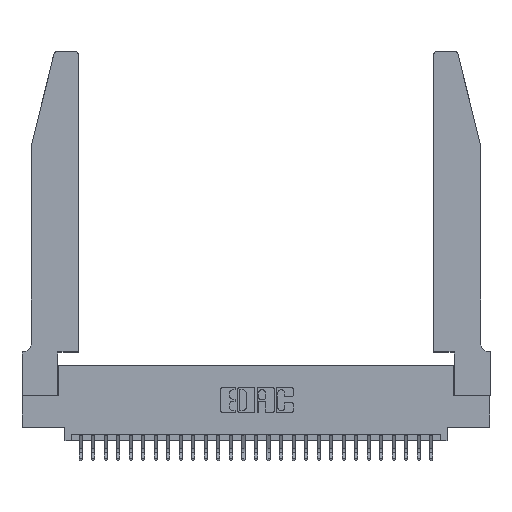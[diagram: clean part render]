
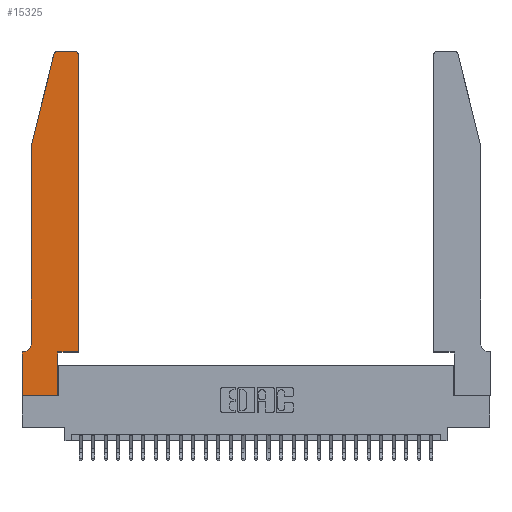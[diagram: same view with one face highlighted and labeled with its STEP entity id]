
A CAD part, top view. The second image highlights one B-rep face of the part: STEP entity #15325.
In plain terms, the highlighted planar face has unit normal (0, 0, 1).
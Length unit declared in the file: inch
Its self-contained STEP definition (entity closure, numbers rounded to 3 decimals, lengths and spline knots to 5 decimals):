
#506 = CARTESIAN_POINT ( 'NONE',  ( 0., 0., 0.37 ) ) ;
#658 = DIRECTION ( 'NONE',  ( -1., 0., 0. ) ) ;
#1285 = VECTOR ( 'NONE', #10921, 39.37008 ) ;
#1309 = ORIENTED_EDGE ( 'NONE', *, *, #6473, .T. ) ;
#1314 = CARTESIAN_POINT ( 'NONE',  ( 0.4505, 0.35, 0.37 ) ) ;
#1376 = CARTESIAN_POINT ( 'NONE',  ( 0., 0.35, 0.37 ) ) ;
#1431 = VECTOR ( 'NONE', #28212, 39.37008 ) ;
#3008 = CARTESIAN_POINT ( 'NONE',  ( 0.4505, 2.72, 0.37 ) ) ;
#3176 = DIRECTION ( 'NONE',  ( 1., 0., 0. ) ) ;
#3518 = VECTOR ( 'NONE', #3176, 39.37008 ) ;
#3612 = DIRECTION ( 'NONE',  ( 0., 1., 0. ) ) ;
#4015 = ORIENTED_EDGE ( 'NONE', *, *, #18248, .T. ) ;
#4120 = DIRECTION ( 'NONE',  ( 0., -1., 0. ) ) ;
#4307 = LINE ( 'NONE', #5317, #1431 ) ;
#5199 = LINE ( 'NONE', #6434, #28792 ) ;
#5227 = CARTESIAN_POINT ( 'NONE',  ( 0.2865, 0.35, 0.37 ) ) ;
#5317 = CARTESIAN_POINT ( 'NONE',  ( 0.0755, 2., 0.37 ) ) ;
#6187 = ORIENTED_EDGE ( 'NONE', *, *, #24921, .T. ) ;
#6309 = CARTESIAN_POINT ( 'NONE',  ( 0., 0.35, 0.37 ) ) ;
#6434 = CARTESIAN_POINT ( 'NONE',  ( 0.0755, 2., 0.37 ) ) ;
#6473 = EDGE_CURVE ( 'NONE', #15882, #16830, #25689, .T. ) ;
#6963 = CIRCLE ( 'NONE', #26165, 0.03 ) ;
#7338 = LINE ( 'NONE', #21954, #19597 ) ;
#7386 = VERTEX_POINT ( 'NONE', #3008 ) ;
#7409 = VERTEX_POINT ( 'NONE', #12400 ) ;
#7676 = EDGE_CURVE ( 'NONE', #7386, #7772, #6963, .T. ) ;
#7711 = CARTESIAN_POINT ( 'NONE',  ( 0.0755, 2., 0.37 ) ) ;
#7722 = ORIENTED_EDGE ( 'NONE', *, *, #14807, .T. ) ;
#7772 = VERTEX_POINT ( 'NONE', #24947 ) ;
#7819 = EDGE_CURVE ( 'NONE', #8067, #19087, #27696, .T. ) ;
#8067 = VERTEX_POINT ( 'NONE', #12265 ) ;
#8667 = DIRECTION ( 'NONE',  ( 0., 0., 1. ) ) ;
#9138 = CARTESIAN_POINT ( 'NONE',  ( 0.4505, 0.35, 0.37 ) ) ;
#10316 = VECTOR ( 'NONE', #17226, 39.37008 ) ;
#10583 = CIRCLE ( 'NONE', #28359, 0.07 ) ;
#10623 = DIRECTION ( 'NONE',  ( 0., 0., 1. ) ) ;
#10705 = ORIENTED_EDGE ( 'NONE', *, *, #15169, .T. ) ;
#10920 = EDGE_CURVE ( 'NONE', #17502, #20826, #27740, .T. ) ;
#10921 = DIRECTION ( 'NONE',  ( 0., -1., 0. ) ) ;
#11044 = CARTESIAN_POINT ( 'NONE',  ( 0.25487, 2.72718, 0.37 ) ) ;
#11061 = DIRECTION ( 'NONE',  ( 0., 0., 1. ) ) ;
#11456 = DIRECTION ( 'NONE',  ( 1., 0., 0. ) ) ;
#11509 = ORIENTED_EDGE ( 'NONE', *, *, #19586, .T. ) ;
#11796 = ORIENTED_EDGE ( 'NONE', *, *, #10920, .T. ) ;
#12265 = CARTESIAN_POINT ( 'NONE',  ( 0.2865, 0.35, 0.37 ) ) ;
#12400 = CARTESIAN_POINT ( 'NONE',  ( 0.2865, 0., 0.37 ) ) ;
#12866 = EDGE_CURVE ( 'NONE', #7409, #8067, #25938, .T. ) ;
#12951 = FACE_OUTER_BOUND ( 'NONE', #21626, .T. ) ;
#13052 = ORIENTED_EDGE ( 'NONE', *, *, #23937, .T. ) ;
#13633 = VERTEX_POINT ( 'NONE', #14590 ) ;
#14269 = VERTEX_POINT ( 'NONE', #21919 ) ;
#14295 = CARTESIAN_POINT ( 'NONE',  ( 0.284, 2.75, 0.37 ) ) ;
#14491 = DIRECTION ( 'NONE',  ( 0., 0., -1. ) ) ;
#14590 = CARTESIAN_POINT ( 'NONE',  ( 0.0755, 0.42, 0.37 ) ) ;
#14689 = CARTESIAN_POINT ( 'NONE',  ( 0., 0., 0.37 ) ) ;
#14807 = EDGE_CURVE ( 'NONE', #20826, #18252, #4307, .T. ) ;
#14914 = VECTOR ( 'NONE', #11456, 39.37008 ) ;
#15169 = EDGE_CURVE ( 'NONE', #19087, #7386, #23322, .T. ) ;
#15325 = ADVANCED_FACE ( 'NONE', ( #12951 ), #20117, .T. ) ;
#15882 = VERTEX_POINT ( 'NONE', #1376 ) ;
#16058 = ORIENTED_EDGE ( 'NONE', *, *, #12866, .T. ) ;
#16565 = VECTOR ( 'NONE', #3612, 39.37008 ) ;
#16591 = ORIENTED_EDGE ( 'NONE', *, *, #28796, .T. ) ;
#16830 = VERTEX_POINT ( 'NONE', #506 ) ;
#17158 = LINE ( 'NONE', #19515, #10316 ) ;
#17226 = DIRECTION ( 'NONE',  ( -1., 0., 0. ) ) ;
#17502 = VERTEX_POINT ( 'NONE', #14295 ) ;
#17649 = CARTESIAN_POINT ( 'NONE',  ( 0., 0., 0.37 ) ) ;
#18248 = EDGE_CURVE ( 'NONE', #16830, #7409, #27143, .T. ) ;
#18252 = VERTEX_POINT ( 'NONE', #7711 ) ;
#19031 = DIRECTION ( 'NONE',  ( 0., 1., 0. ) ) ;
#19087 = VERTEX_POINT ( 'NONE', #26840 ) ;
#19515 = CARTESIAN_POINT ( 'NONE',  ( 0.2605, 2.75, 0.37 ) ) ;
#19586 = EDGE_CURVE ( 'NONE', #7772, #17502, #17158, .T. ) ;
#19597 = VECTOR ( 'NONE', #21855, 39.37008 ) ;
#19903 = VECTOR ( 'NONE', #19031, 39.37008 ) ;
#20117 = PLANE ( 'NONE',  #26287 ) ;
#20826 = VERTEX_POINT ( 'NONE', #11044 ) ;
#21493 = ORIENTED_EDGE ( 'NONE', *, *, #7819, .T. ) ;
#21626 = EDGE_LOOP ( 'NONE', ( #11509, #11796, #7722, #13052, #6187, #16591, #1309, #4015, #16058, #21493, #10705, #26488 ) ) ;
#21855 = DIRECTION ( 'NONE',  ( -1., 0., 0. ) ) ;
#21919 = CARTESIAN_POINT ( 'NONE',  ( 0.0055, 0.35, 0.37 ) ) ;
#21954 = CARTESIAN_POINT ( 'NONE',  ( 0.0755, 0.35, 0.37 ) ) ;
#22590 = AXIS2_PLACEMENT_3D ( 'NONE', #24313, #10623, #26570 ) ;
#23322 = LINE ( 'NONE', #1314, #16565 ) ;
#23937 = EDGE_CURVE ( 'NONE', #18252, #13633, #5199, .T. ) ;
#24313 = CARTESIAN_POINT ( 'NONE',  ( 0.284, 2.72, 0.37 ) ) ;
#24683 = DIRECTION ( 'NONE',  ( 1., 0., 0. ) ) ;
#24756 = CARTESIAN_POINT ( 'NONE',  ( 0.4205, 2.72, 0.37 ) ) ;
#24921 = EDGE_CURVE ( 'NONE', #13633, #14269, #10583, .T. ) ;
#24947 = CARTESIAN_POINT ( 'NONE',  ( 0.4205, 2.75, 0.37 ) ) ;
#25689 = LINE ( 'NONE', #17649, #1285 ) ;
#25938 = LINE ( 'NONE', #5227, #19903 ) ;
#26165 = AXIS2_PLACEMENT_3D ( 'NONE', #24756, #11061, #26994 ) ;
#26287 = AXIS2_PLACEMENT_3D ( 'NONE', #6309, #8667, #24683 ) ;
#26488 = ORIENTED_EDGE ( 'NONE', *, *, #7676, .T. ) ;
#26570 = DIRECTION ( 'NONE',  ( 1., 0., 0. ) ) ;
#26840 = CARTESIAN_POINT ( 'NONE',  ( 0.4505, 0.35, 0.37 ) ) ;
#26994 = DIRECTION ( 'NONE',  ( 1., 0., 0. ) ) ;
#27143 = LINE ( 'NONE', #14689, #3518 ) ;
#27696 = LINE ( 'NONE', #9138, #14914 ) ;
#27740 = CIRCLE ( 'NONE', #22590, 0.03 ) ;
#28073 = CARTESIAN_POINT ( 'NONE',  ( 0.0055, 0.42, 0.37 ) ) ;
#28212 = DIRECTION ( 'NONE',  ( -0.239, -0.971, 0. ) ) ;
#28359 = AXIS2_PLACEMENT_3D ( 'NONE', #28073, #14491, #658 ) ;
#28792 = VECTOR ( 'NONE', #4120, 39.37008 ) ;
#28796 = EDGE_CURVE ( 'NONE', #14269, #15882, #7338, .T. ) ;
